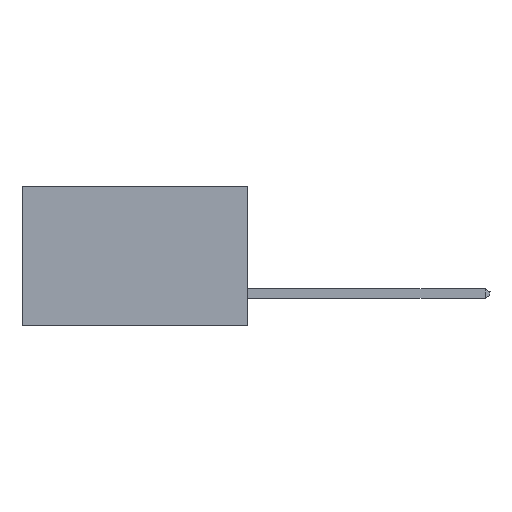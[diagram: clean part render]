
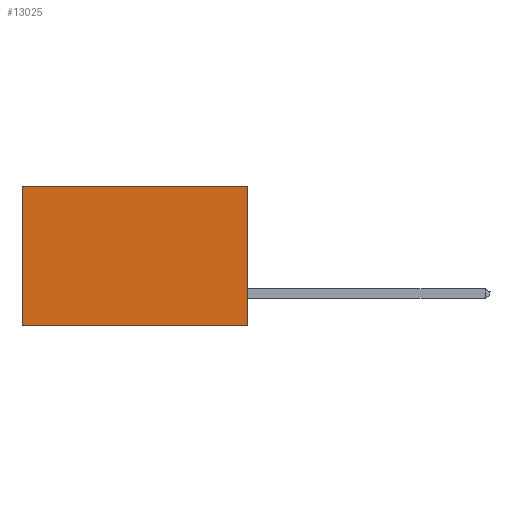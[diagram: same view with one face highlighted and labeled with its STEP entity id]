
A CAD part, left-side view. The second image highlights one B-rep face of the part: STEP entity #13025.
In plain terms, the highlighted planar face has unit normal (-1, 0, 0).
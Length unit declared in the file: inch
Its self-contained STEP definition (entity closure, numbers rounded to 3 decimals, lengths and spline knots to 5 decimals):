
#134 = ORIENTED_EDGE ( 'NONE', *, *, #4735, .T. ) ;
#482 = EDGE_CURVE ( 'NONE', #13265, #13446, #11685, .T. ) ;
#741 = EDGE_CURVE ( 'NONE', #7384, #9369, #10964, .T. ) ;
#1041 = ORIENTED_EDGE ( 'NONE', *, *, #482, .T. ) ;
#1765 = VECTOR ( 'NONE', #16075, 39.37008 ) ;
#1841 = CARTESIAN_POINT ( 'NONE',  ( 0.2615, 0., -0.37 ) ) ;
#2329 = CARTESIAN_POINT ( 'NONE',  ( 0.2615, 0., -0.37 ) ) ;
#2451 = EDGE_LOOP ( 'NONE', ( #1041, #17382, #10355, #134 ) ) ;
#3399 = LINE ( 'NONE', #2329, #5834 ) ;
#3432 = CARTESIAN_POINT ( 'NONE',  ( 0.2615, 0.6, -0.37 ) ) ;
#3578 = CARTESIAN_POINT ( 'NONE',  ( 0.2615, 0.6, -0.37 ) ) ;
#4735 = EDGE_CURVE ( 'NONE', #7384, #13265, #7830, .T. ) ;
#5834 = VECTOR ( 'NONE', #6269, 39.37008 ) ;
#6066 = PLANE ( 'NONE',  #7652 ) ;
#6130 = DIRECTION ( 'NONE',  ( 0., 0., -1. ) ) ;
#6158 = DIRECTION ( 'NONE',  ( 0., 0., -1. ) ) ;
#6269 = DIRECTION ( 'NONE',  ( 0., 1., 0. ) ) ;
#7098 = CARTESIAN_POINT ( 'NONE',  ( 0.2615, 0., -0.37 ) ) ;
#7231 = CARTESIAN_POINT ( 'NONE',  ( 0.2615, 0., -0.37 ) ) ;
#7384 = VERTEX_POINT ( 'NONE', #7720 ) ;
#7652 = AXIS2_PLACEMENT_3D ( 'NONE', #7231, #14230, #6158 ) ;
#7703 = EDGE_CURVE ( 'NONE', #9369, #13446, #3399, .T. ) ;
#7720 = CARTESIAN_POINT ( 'NONE',  ( 0.2615, 0., 0. ) ) ;
#7830 = LINE ( 'NONE', #14552, #1765 ) ;
#8838 = FACE_OUTER_BOUND ( 'NONE', #2451, .T. ) ;
#9369 = VERTEX_POINT ( 'NONE', #1841 ) ;
#10355 = ORIENTED_EDGE ( 'NONE', *, *, #741, .F. ) ;
#10964 = LINE ( 'NONE', #7098, #11154 ) ;
#11154 = VECTOR ( 'NONE', #15260, 39.37008 ) ;
#11685 = LINE ( 'NONE', #3432, #15104 ) ;
#12623 = CARTESIAN_POINT ( 'NONE',  ( 0.2615, 0.6, 0. ) ) ;
#13025 = ADVANCED_FACE ( 'NONE', ( #8838 ), #6066, .F. ) ;
#13265 = VERTEX_POINT ( 'NONE', #12623 ) ;
#13446 = VERTEX_POINT ( 'NONE', #3578 ) ;
#14230 = DIRECTION ( 'NONE',  ( 1., 0., 0. ) ) ;
#14552 = CARTESIAN_POINT ( 'NONE',  ( 0.2615, 0., 0. ) ) ;
#15104 = VECTOR ( 'NONE', #6130, 39.37008 ) ;
#15260 = DIRECTION ( 'NONE',  ( 0., 0., -1. ) ) ;
#16075 = DIRECTION ( 'NONE',  ( 0., 1., 0. ) ) ;
#17382 = ORIENTED_EDGE ( 'NONE', *, *, #7703, .F. ) ;
